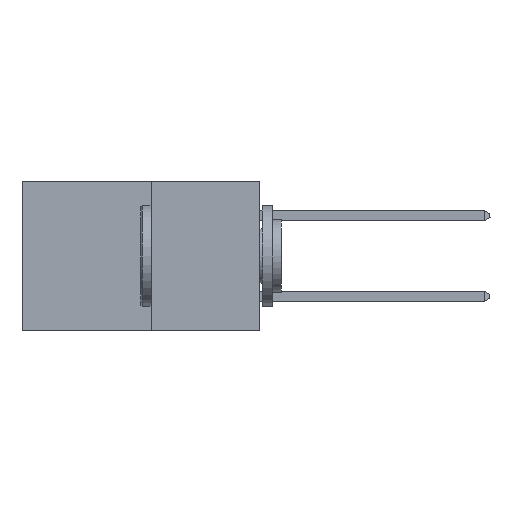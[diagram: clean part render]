
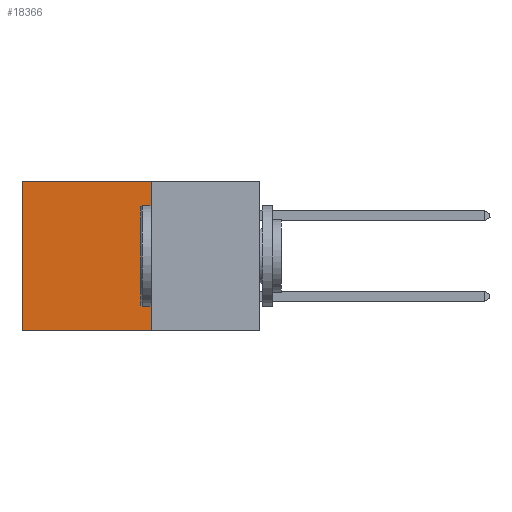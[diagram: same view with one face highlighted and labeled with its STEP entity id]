
A CAD part, left-side view. The second image highlights one B-rep face of the part: STEP entity #18366.
In plain terms, the highlighted planar face has unit normal (-1, 0, 0).
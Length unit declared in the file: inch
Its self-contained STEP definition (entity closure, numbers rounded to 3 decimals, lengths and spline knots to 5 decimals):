
#1644 = ORIENTED_EDGE ( 'NONE', *, *, #14131, .F. ) ;
#2085 = ORIENTED_EDGE ( 'NONE', *, *, #33319, .T. ) ;
#3701 = CARTESIAN_POINT ( 'NONE',  ( 0.277, 0.59, -0.37 ) ) ;
#3894 = CARTESIAN_POINT ( 'NONE',  ( 0.277, 0.59, -0.37 ) ) ;
#3940 = CARTESIAN_POINT ( 'NONE',  ( 0.277, 0.27, -0.37 ) ) ;
#7347 = CARTESIAN_POINT ( 'NONE',  ( 0.277, 0.27, -0.37 ) ) ;
#8859 = AXIS2_PLACEMENT_3D ( 'NONE', #3940, #11950, #30509 ) ;
#9633 = ORIENTED_EDGE ( 'NONE', *, *, #14556, .F. ) ;
#9684 = CARTESIAN_POINT ( 'NONE',  ( 0.277, 0.27, -0.37 ) ) ;
#10410 = VECTOR ( 'NONE', #29849, 39.37008 ) ;
#11950 = DIRECTION ( 'NONE',  ( 1., 0., 0. ) ) ;
#12062 = LINE ( 'NONE', #21490, #10410 ) ;
#12151 = VECTOR ( 'NONE', #22262, 39.37008 ) ;
#12328 = DIRECTION ( 'NONE',  ( 0., 1., 0. ) ) ;
#14131 = EDGE_CURVE ( 'NONE', #26674, #21096, #19058, .T. ) ;
#14556 = EDGE_CURVE ( 'NONE', #21096, #32843, #19852, .T. ) ;
#18366 = ADVANCED_FACE ( 'NONE', ( #28122 ), #27821, .F. ) ;
#19058 = LINE ( 'NONE', #21018, #25260 ) ;
#19451 = ORIENTED_EDGE ( 'NONE', *, *, #22284, .T. ) ;
#19852 = LINE ( 'NONE', #9684, #26054 ) ;
#21018 = CARTESIAN_POINT ( 'NONE',  ( 0.277, 0.27, -0.37 ) ) ;
#21096 = VERTEX_POINT ( 'NONE', #7347 ) ;
#21362 = CARTESIAN_POINT ( 'NONE',  ( 0.277, 0.27, 0. ) ) ;
#21490 = CARTESIAN_POINT ( 'NONE',  ( 0.277, 0.27, 0. ) ) ;
#21895 = EDGE_LOOP ( 'NONE', ( #19451, #9633, #1644, #2085 ) ) ;
#22262 = DIRECTION ( 'NONE',  ( 0., 0., -1. ) ) ;
#22284 = EDGE_CURVE ( 'NONE', #33055, #32843, #27055, .T. ) ;
#23662 = DIRECTION ( 'NONE',  ( 0., 0., -1. ) ) ;
#25260 = VECTOR ( 'NONE', #23662, 39.37008 ) ;
#26054 = VECTOR ( 'NONE', #12328, 39.37008 ) ;
#26674 = VERTEX_POINT ( 'NONE', #21362 ) ;
#27055 = LINE ( 'NONE', #3701, #12151 ) ;
#27821 = PLANE ( 'NONE',  #8859 ) ;
#28122 = FACE_OUTER_BOUND ( 'NONE', #21895, .T. ) ;
#28563 = CARTESIAN_POINT ( 'NONE',  ( 0.277, 0.59, 0. ) ) ;
#29849 = DIRECTION ( 'NONE',  ( 0., 1., 0. ) ) ;
#30509 = DIRECTION ( 'NONE',  ( 0., 0., -1. ) ) ;
#32843 = VERTEX_POINT ( 'NONE', #3894 ) ;
#33055 = VERTEX_POINT ( 'NONE', #28563 ) ;
#33319 = EDGE_CURVE ( 'NONE', #26674, #33055, #12062, .T. ) ;
